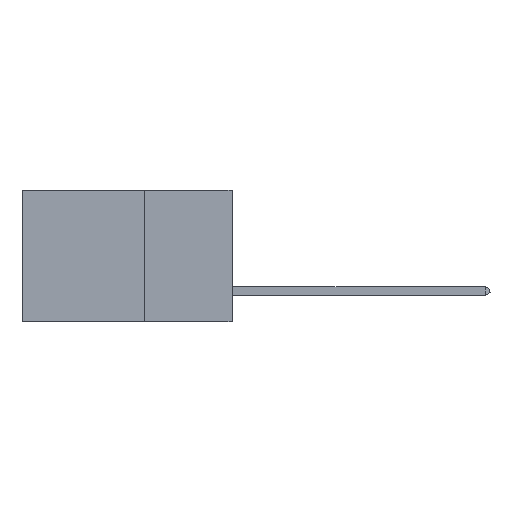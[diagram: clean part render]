
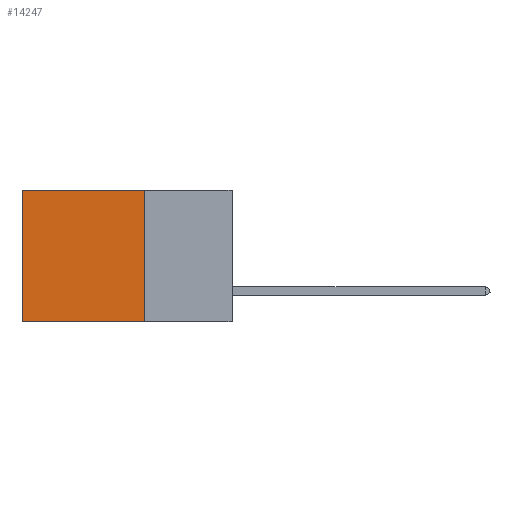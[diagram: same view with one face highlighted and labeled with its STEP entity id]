
A CAD part, left-side view. The second image highlights one B-rep face of the part: STEP entity #14247.
In plain terms, the highlighted planar face has unit normal (-1, 0, 0).
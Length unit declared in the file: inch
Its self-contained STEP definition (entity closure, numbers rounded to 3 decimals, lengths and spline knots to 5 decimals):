
#1374 = VECTOR ( 'NONE', #15852, 39.37008 ) ;
#1654 = CARTESIAN_POINT ( 'NONE',  ( 0.2875, 0.25, -0.375 ) ) ;
#1801 = VECTOR ( 'NONE', #16190, 39.37008 ) ;
#2144 = CARTESIAN_POINT ( 'NONE',  ( 0.2875, 0.25, 0. ) ) ;
#3424 = PLANE ( 'NONE',  #19228 ) ;
#4033 = LINE ( 'NONE', #2144, #1374 ) ;
#4044 = FACE_OUTER_BOUND ( 'NONE', #17630, .T. ) ;
#4910 = DIRECTION ( 'NONE',  ( 0., 0., -1. ) ) ;
#5425 = CARTESIAN_POINT ( 'NONE',  ( 0.2875, 0.6, 0. ) ) ;
#6657 = VERTEX_POINT ( 'NONE', #20498 ) ;
#9057 = ORIENTED_EDGE ( 'NONE', *, *, #18807, .T. ) ;
#10127 = CARTESIAN_POINT ( 'NONE',  ( 0.2875, 0.25, -0.375 ) ) ;
#10227 = CARTESIAN_POINT ( 'NONE',  ( 0.2875, 0.6, -0.375 ) ) ;
#10309 = EDGE_CURVE ( 'NONE', #12668, #6657, #13116, .T. ) ;
#11289 = ORIENTED_EDGE ( 'NONE', *, *, #21707, .F. ) ;
#12319 = ORIENTED_EDGE ( 'NONE', *, *, #19441, .T. ) ;
#12668 = VERTEX_POINT ( 'NONE', #18539 ) ;
#12820 = VERTEX_POINT ( 'NONE', #5425 ) ;
#13116 = LINE ( 'NONE', #19317, #1801 ) ;
#13338 = LINE ( 'NONE', #1654, #20219 ) ;
#13355 = DIRECTION ( 'NONE',  ( 0., 1., 0. ) ) ;
#14247 = ADVANCED_FACE ( 'NONE', ( #4044 ), #3424, .F. ) ;
#15001 = ORIENTED_EDGE ( 'NONE', *, *, #10309, .F. ) ;
#15553 = VERTEX_POINT ( 'NONE', #15923 ) ;
#15852 = DIRECTION ( 'NONE',  ( 0., 1., 0. ) ) ;
#15923 = CARTESIAN_POINT ( 'NONE',  ( 0.2875, 0.6, -0.375 ) ) ;
#16190 = DIRECTION ( 'NONE',  ( 0., 0., -1. ) ) ;
#17630 = EDGE_LOOP ( 'NONE', ( #12319, #11289, #15001, #9057 ) ) ;
#18539 = CARTESIAN_POINT ( 'NONE',  ( 0.2875, 0.25, 0. ) ) ;
#18807 = EDGE_CURVE ( 'NONE', #12668, #12820, #4033, .T. ) ;
#19042 = LINE ( 'NONE', #10227, #20868 ) ;
#19228 = AXIS2_PLACEMENT_3D ( 'NONE', #10127, #20164, #4910 ) ;
#19317 = CARTESIAN_POINT ( 'NONE',  ( 0.2875, 0.25, -0.375 ) ) ;
#19441 = EDGE_CURVE ( 'NONE', #12820, #15553, #19042, .T. ) ;
#20164 = DIRECTION ( 'NONE',  ( 1., 0., 0. ) ) ;
#20219 = VECTOR ( 'NONE', #13355, 39.37008 ) ;
#20399 = DIRECTION ( 'NONE',  ( 0., 0., -1. ) ) ;
#20498 = CARTESIAN_POINT ( 'NONE',  ( 0.2875, 0.25, -0.375 ) ) ;
#20868 = VECTOR ( 'NONE', #20399, 39.37008 ) ;
#21707 = EDGE_CURVE ( 'NONE', #6657, #15553, #13338, .T. ) ;
